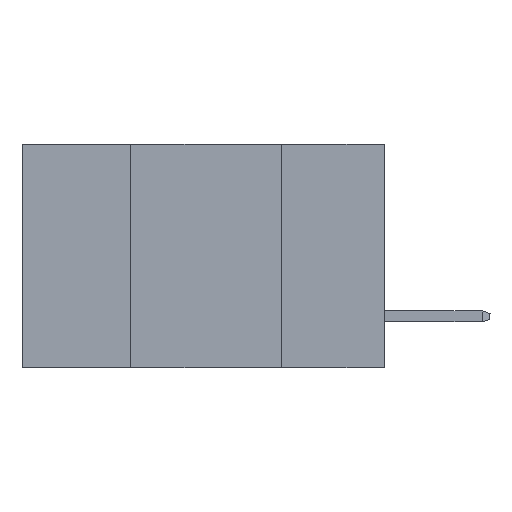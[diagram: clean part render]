
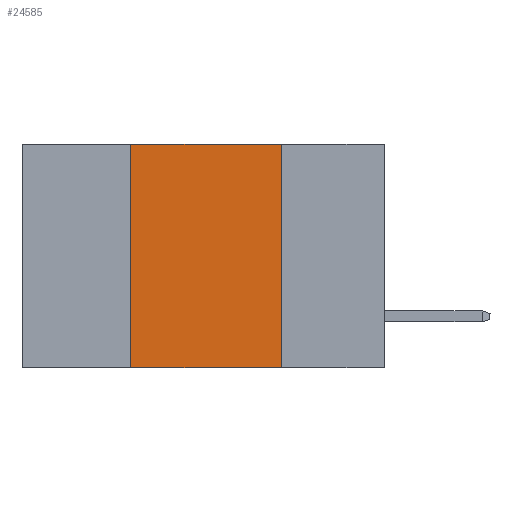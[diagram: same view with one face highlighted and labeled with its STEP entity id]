
A CAD part, left-side view. The second image highlights one B-rep face of the part: STEP entity #24585.
In plain terms, the highlighted planar face has unit normal (-1, 0, 0).
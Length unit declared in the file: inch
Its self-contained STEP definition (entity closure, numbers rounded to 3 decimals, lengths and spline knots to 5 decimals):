
#508 = EDGE_CURVE ( 'NONE', #8827, #6293, #7560, .T. ) ;
#550 = CARTESIAN_POINT ( 'NONE',  ( 0., 0.17, -0.37 ) ) ;
#621 = VECTOR ( 'NONE', #13777, 39.37008 ) ;
#1390 = LINE ( 'NONE', #17624, #2446 ) ;
#2446 = VECTOR ( 'NONE', #5287, 39.37008 ) ;
#4113 = CARTESIAN_POINT ( 'NONE',  ( 0., 0.42, 0. ) ) ;
#4775 = CARTESIAN_POINT ( 'NONE',  ( 0., 0.6, 0. ) ) ;
#5234 = ORIENTED_EDGE ( 'NONE', *, *, #5465, .T. ) ;
#5287 = DIRECTION ( 'NONE',  ( 0., -1., 0. ) ) ;
#5465 = EDGE_CURVE ( 'NONE', #16714, #20687, #1390, .T. ) ;
#5588 = CARTESIAN_POINT ( 'NONE',  ( 0., 0.17, 0. ) ) ;
#6293 = VERTEX_POINT ( 'NONE', #5588 ) ;
#6811 = CARTESIAN_POINT ( 'NONE',  ( 0., 0.42, -0.37 ) ) ;
#7423 = CARTESIAN_POINT ( 'NONE',  ( 0., 0.42, -0.37 ) ) ;
#7560 = LINE ( 'NONE', #19740, #621 ) ;
#8827 = VERTEX_POINT ( 'NONE', #4113 ) ;
#9161 = ORIENTED_EDGE ( 'NONE', *, *, #13616, .F. ) ;
#10502 = PLANE ( 'NONE',  #19420 ) ;
#11477 = VECTOR ( 'NONE', #20285, 39.37008 ) ;
#13616 = EDGE_CURVE ( 'NONE', #16714, #8827, #17292, .T. ) ;
#13777 = DIRECTION ( 'NONE',  ( 0., -1., 0. ) ) ;
#14799 = FACE_OUTER_BOUND ( 'NONE', #22798, .T. ) ;
#15340 = DIRECTION ( 'NONE',  ( 0., 0., 1. ) ) ;
#15443 = VECTOR ( 'NONE', #15340, 39.37008 ) ;
#15893 = LINE ( 'NONE', #550, #11477 ) ;
#16714 = VERTEX_POINT ( 'NONE', #6811 ) ;
#17292 = LINE ( 'NONE', #7423, #15443 ) ;
#17624 = CARTESIAN_POINT ( 'NONE',  ( 0., 0.6, -0.37 ) ) ;
#18424 = DIRECTION ( 'NONE',  ( 1., 0., 0. ) ) ;
#19420 = AXIS2_PLACEMENT_3D ( 'NONE', #4775, #18424, #22678 ) ;
#19740 = CARTESIAN_POINT ( 'NONE',  ( 0., 0.6, 0. ) ) ;
#20285 = DIRECTION ( 'NONE',  ( 0., 0., -1. ) ) ;
#20687 = VERTEX_POINT ( 'NONE', #21579 ) ;
#21438 = ORIENTED_EDGE ( 'NONE', *, *, #22243, .F. ) ;
#21579 = CARTESIAN_POINT ( 'NONE',  ( 0., 0.17, -0.37 ) ) ;
#21587 = ORIENTED_EDGE ( 'NONE', *, *, #508, .F. ) ;
#22243 = EDGE_CURVE ( 'NONE', #6293, #20687, #15893, .T. ) ;
#22678 = DIRECTION ( 'NONE',  ( 0., 0., -1. ) ) ;
#22798 = EDGE_LOOP ( 'NONE', ( #21438, #21587, #9161, #5234 ) ) ;
#24585 = ADVANCED_FACE ( 'NONE', ( #14799 ), #10502, .F. ) ;
